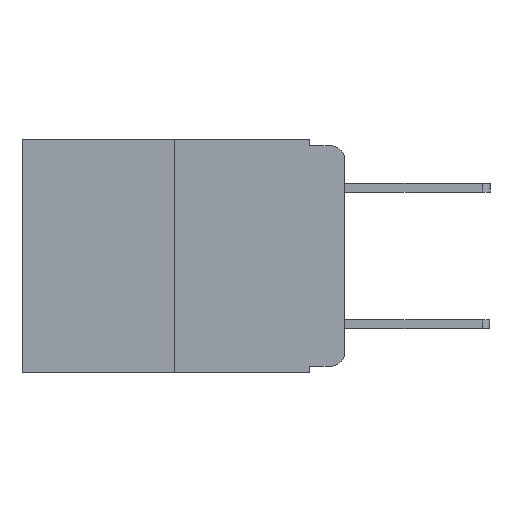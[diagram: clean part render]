
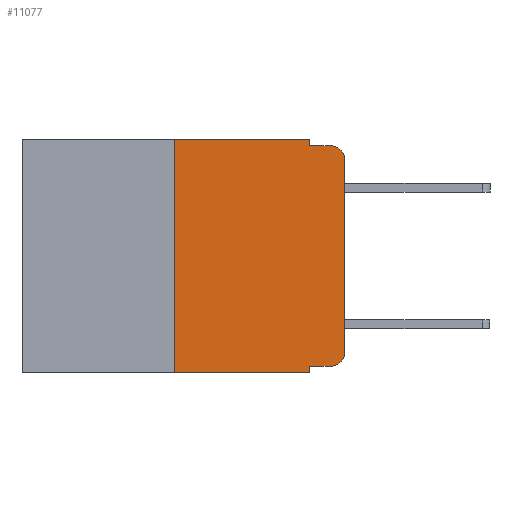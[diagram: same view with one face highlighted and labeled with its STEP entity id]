
A CAD part, left-side view. The second image highlights one B-rep face of the part: STEP entity #11077.
In plain terms, the highlighted planar face has unit normal (-1, 0, 0).
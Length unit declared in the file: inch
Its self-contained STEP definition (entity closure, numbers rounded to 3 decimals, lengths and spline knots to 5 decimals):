
#312 = DIRECTION ( 'NONE',  ( 0., 0., -1. ) ) ;
#390 = VERTEX_POINT ( 'NONE', #24644 ) ;
#1169 = ORIENTED_EDGE ( 'NONE', *, *, #11366, .T. ) ;
#1792 = ORIENTED_EDGE ( 'NONE', *, *, #2543, .T. ) ;
#2026 = EDGE_CURVE ( 'NONE', #8254, #10182, #22703, .T. ) ;
#2543 = EDGE_CURVE ( 'NONE', #5474, #23925, #9618, .T. ) ;
#2747 = CARTESIAN_POINT ( 'NONE',  ( 0., 0.25, 0. ) ) ;
#2792 = VERTEX_POINT ( 'NONE', #11001 ) ;
#3751 = CARTESIAN_POINT ( 'NONE',  ( 0., 0.051, -0.01 ) ) ;
#3754 = ORIENTED_EDGE ( 'NONE', *, *, #18324, .F. ) ;
#3949 = VERTEX_POINT ( 'NONE', #3751 ) ;
#4120 = FACE_OUTER_BOUND ( 'NONE', #18638, .T. ) ;
#5129 = CARTESIAN_POINT ( 'NONE',  ( 0., 0.051, 0. ) ) ;
#5145 = CARTESIAN_POINT ( 'NONE',  ( 0., 0.051, -0.333 ) ) ;
#5338 = VECTOR ( 'NONE', #20156, 39.37008 ) ;
#5388 = ORIENTED_EDGE ( 'NONE', *, *, #19138, .T. ) ;
#5395 = DIRECTION ( 'NONE',  ( 0., 0., -1. ) ) ;
#5412 = DIRECTION ( 'NONE',  ( -1., 0., 0. ) ) ;
#5417 = CARTESIAN_POINT ( 'NONE',  ( 0., 0.02, -0.03 ) ) ;
#5474 = VERTEX_POINT ( 'NONE', #16166 ) ;
#5743 = AXIS2_PLACEMENT_3D ( 'NONE', #23111, #11570, #25006 ) ;
#6056 = LINE ( 'NONE', #6559, #25372 ) ;
#6559 = CARTESIAN_POINT ( 'NONE',  ( 0., 0.051, -0.01 ) ) ;
#6693 = VECTOR ( 'NONE', #7087, 39.37008 ) ;
#7087 = DIRECTION ( 'NONE',  ( 0., -1., 0. ) ) ;
#7437 = EDGE_CURVE ( 'NONE', #7786, #22237, #22382, .T. ) ;
#7786 = VERTEX_POINT ( 'NONE', #9686 ) ;
#8254 = VERTEX_POINT ( 'NONE', #24581 ) ;
#9330 = ORIENTED_EDGE ( 'NONE', *, *, #2026, .F. ) ;
#9618 = CIRCLE ( 'NONE', #11654, 0.02 ) ;
#9651 = CARTESIAN_POINT ( 'NONE',  ( 0., 0.051, 0. ) ) ;
#9686 = CARTESIAN_POINT ( 'NONE',  ( 0., 0.25, -0.343 ) ) ;
#9795 = LINE ( 'NONE', #10931, #15566 ) ;
#9893 = EDGE_CURVE ( 'NONE', #22237, #22461, #20896, .T. ) ;
#10096 = VECTOR ( 'NONE', #14196, 39.37008 ) ;
#10182 = VERTEX_POINT ( 'NONE', #21143 ) ;
#10354 = CARTESIAN_POINT ( 'NONE',  ( 0., 0.473, 0. ) ) ;
#10841 = ORIENTED_EDGE ( 'NONE', *, *, #9893, .F. ) ;
#10931 = CARTESIAN_POINT ( 'NONE',  ( 0., 0.473, -0.343 ) ) ;
#11001 = CARTESIAN_POINT ( 'NONE',  ( 0., 0.02, -0.333 ) ) ;
#11077 = ADVANCED_FACE ( 'NONE', ( #4120 ), #21930, .F. ) ;
#11366 = EDGE_CURVE ( 'NONE', #2792, #390, #12408, .T. ) ;
#11479 = AXIS2_PLACEMENT_3D ( 'NONE', #10354, #12334, #312 ) ;
#11570 = DIRECTION ( 'NONE',  ( -1., 0., 0. ) ) ;
#11654 = AXIS2_PLACEMENT_3D ( 'NONE', #5417, #5412, #5395 ) ;
#12138 = VECTOR ( 'NONE', #24122, 39.37008 ) ;
#12262 = CARTESIAN_POINT ( 'NONE',  ( 0., 0.051, 0. ) ) ;
#12309 = CARTESIAN_POINT ( 'NONE',  ( 0., 0.25, 0. ) ) ;
#12334 = DIRECTION ( 'NONE',  ( 1., 0., 0. ) ) ;
#12360 = EDGE_CURVE ( 'NONE', #390, #5474, #20814, .T. ) ;
#12397 = CARTESIAN_POINT ( 'NONE',  ( 0., 0., 0. ) ) ;
#12408 = CIRCLE ( 'NONE', #5743, 0.02 ) ;
#12474 = CARTESIAN_POINT ( 'NONE',  ( 0., 0.473, 0. ) ) ;
#12997 = ORIENTED_EDGE ( 'NONE', *, *, #19636, .F. ) ;
#14191 = EDGE_CURVE ( 'NONE', #7786, #10182, #9795, .T. ) ;
#14196 = DIRECTION ( 'NONE',  ( 0., 0., -1. ) ) ;
#14314 = DIRECTION ( 'NONE',  ( 0., -1., 0. ) ) ;
#14407 = DIRECTION ( 'NONE',  ( 0., -1., 0. ) ) ;
#15088 = ORIENTED_EDGE ( 'NONE', *, *, #12360, .T. ) ;
#15566 = VECTOR ( 'NONE', #24408, 39.37008 ) ;
#15755 = VECTOR ( 'NONE', #14407, 39.37008 ) ;
#16166 = CARTESIAN_POINT ( 'NONE',  ( 0., 0., -0.03 ) ) ;
#17048 = LINE ( 'NONE', #5145, #6693 ) ;
#17602 = DIRECTION ( 'NONE',  ( 0., 0., -1. ) ) ;
#18102 = LINE ( 'NONE', #12262, #10096 ) ;
#18324 = EDGE_CURVE ( 'NONE', #22461, #3949, #18102, .T. ) ;
#18638 = EDGE_LOOP ( 'NONE', ( #15088, #1792, #12997, #3754, #10841, #22331, #22937, #9330, #5388, #1169 ) ) ;
#19138 = EDGE_CURVE ( 'NONE', #8254, #2792, #17048, .T. ) ;
#19636 = EDGE_CURVE ( 'NONE', #3949, #23925, #6056, .T. ) ;
#20156 = DIRECTION ( 'NONE',  ( 0., 0., 1. ) ) ;
#20814 = LINE ( 'NONE', #12397, #5338 ) ;
#20896 = LINE ( 'NONE', #12474, #15755 ) ;
#21143 = CARTESIAN_POINT ( 'NONE',  ( 0., 0.051, -0.343 ) ) ;
#21930 = PLANE ( 'NONE',  #11479 ) ;
#22099 = VECTOR ( 'NONE', #17602, 39.37008 ) ;
#22237 = VERTEX_POINT ( 'NONE', #12309 ) ;
#22331 = ORIENTED_EDGE ( 'NONE', *, *, #7437, .F. ) ;
#22382 = LINE ( 'NONE', #2747, #12138 ) ;
#22461 = VERTEX_POINT ( 'NONE', #5129 ) ;
#22703 = LINE ( 'NONE', #9651, #22099 ) ;
#22937 = ORIENTED_EDGE ( 'NONE', *, *, #14191, .T. ) ;
#23111 = CARTESIAN_POINT ( 'NONE',  ( 0., 0.02, -0.313 ) ) ;
#23449 = CARTESIAN_POINT ( 'NONE',  ( 0., 0.02, -0.01 ) ) ;
#23925 = VERTEX_POINT ( 'NONE', #23449 ) ;
#24122 = DIRECTION ( 'NONE',  ( 0., 0., 1. ) ) ;
#24408 = DIRECTION ( 'NONE',  ( 0., -1., 0. ) ) ;
#24581 = CARTESIAN_POINT ( 'NONE',  ( 0., 0.051, -0.333 ) ) ;
#24644 = CARTESIAN_POINT ( 'NONE',  ( 0., 0., -0.313 ) ) ;
#25006 = DIRECTION ( 'NONE',  ( 0., 0., -1. ) ) ;
#25372 = VECTOR ( 'NONE', #14314, 39.37008 ) ;
